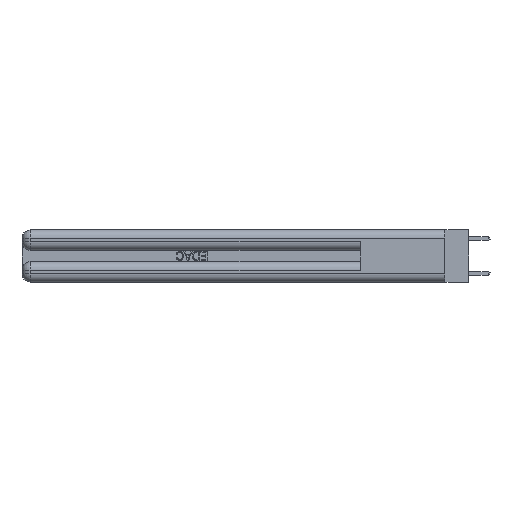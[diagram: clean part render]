
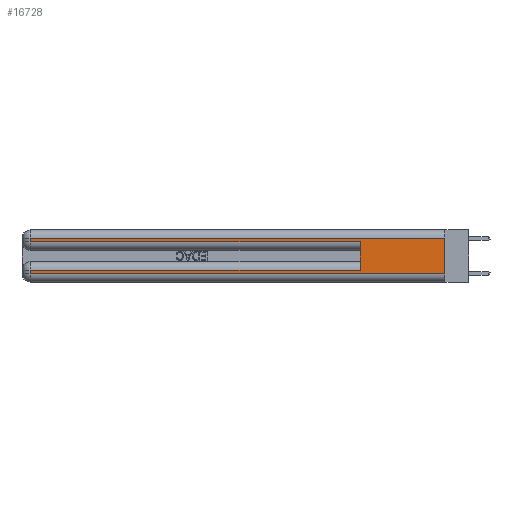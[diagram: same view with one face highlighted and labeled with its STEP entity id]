
A CAD part, left-side view. The second image highlights one B-rep face of the part: STEP entity #16728.
In plain terms, the highlighted planar face has unit normal (-1, 0, 0).
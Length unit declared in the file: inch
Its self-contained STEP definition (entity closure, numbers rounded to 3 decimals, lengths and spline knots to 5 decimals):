
#50 = CARTESIAN_POINT ( 'NONE',  ( 0., 0., 0.285 ) ) ;
#538 = DIRECTION ( 'NONE',  ( 0., 0., 1. ) ) ;
#774 = FACE_OUTER_BOUND ( 'NONE', #30095, .T. ) ;
#947 = VECTOR ( 'NONE', #8638, 39.37008 ) ;
#1196 = EDGE_CURVE ( 'NONE', #1307, #21893, #12783, .T. ) ;
#1307 = VERTEX_POINT ( 'NONE', #31573 ) ;
#3032 = CARTESIAN_POINT ( 'NONE',  ( 0., 0., 0.31 ) ) ;
#3648 = VERTEX_POINT ( 'NONE', #25622 ) ;
#3710 = CARTESIAN_POINT ( 'NONE',  ( 0., 0., 0.37 ) ) ;
#3762 = CARTESIAN_POINT ( 'NONE',  ( 0., 0.6, 0.145 ) ) ;
#4856 = EDGE_CURVE ( 'NONE', #10565, #1307, #28191, .T. ) ;
#5400 = DIRECTION ( 'NONE',  ( 1., 0., 0. ) ) ;
#6065 = CARTESIAN_POINT ( 'NONE',  ( 0., 0., 0.37 ) ) ;
#6558 = CARTESIAN_POINT ( 'NONE',  ( 0., 2.94, 0.31 ) ) ;
#6879 = CARTESIAN_POINT ( 'NONE',  ( 0., 0., 0.31 ) ) ;
#7397 = EDGE_CURVE ( 'NONE', #10565, #8087, #21836, .T. ) ;
#8087 = VERTEX_POINT ( 'NONE', #17876 ) ;
#8638 = DIRECTION ( 'NONE',  ( 0., -1., 0. ) ) ;
#9227 = ORIENTED_EDGE ( 'NONE', *, *, #4856, .T. ) ;
#10565 = VERTEX_POINT ( 'NONE', #12717 ) ;
#12412 = AXIS2_PLACEMENT_3D ( 'NONE', #6065, #5400, #16480 ) ;
#12717 = CARTESIAN_POINT ( 'NONE',  ( 0., 0.6, 0.085 ) ) ;
#12783 = LINE ( 'NONE', #18262, #14781 ) ;
#13610 = LINE ( 'NONE', #21123, #947 ) ;
#14781 = VECTOR ( 'NONE', #20474, 39.37008 ) ;
#15337 = EDGE_CURVE ( 'NONE', #31541, #3648, #23292, .T. ) ;
#15929 = CARTESIAN_POINT ( 'NONE',  ( 0., 2.94, 0.06 ) ) ;
#16176 = VECTOR ( 'NONE', #23125, 39.37008 ) ;
#16387 = EDGE_CURVE ( 'NONE', #21893, #32564, #13610, .T. ) ;
#16480 = DIRECTION ( 'NONE',  ( 0., 0., -1. ) ) ;
#16561 = CARTESIAN_POINT ( 'NONE',  ( 0., 0., 0.06 ) ) ;
#16728 = ADVANCED_FACE ( 'NONE', ( #774 ), #23965, .F. ) ;
#16973 = VECTOR ( 'NONE', #24961, 39.37008 ) ;
#17876 = CARTESIAN_POINT ( 'NONE',  ( 0., 0.6, 0.285 ) ) ;
#17976 = ORIENTED_EDGE ( 'NONE', *, *, #20560, .T. ) ;
#18227 = VECTOR ( 'NONE', #27723, 39.37008 ) ;
#18262 = CARTESIAN_POINT ( 'NONE',  ( 0., 2.94, 0.37 ) ) ;
#18801 = ORIENTED_EDGE ( 'NONE', *, *, #7397, .F. ) ;
#20187 = CARTESIAN_POINT ( 'NONE',  ( 0., 0., 0.085 ) ) ;
#20474 = DIRECTION ( 'NONE',  ( 0., 0., -1. ) ) ;
#20560 = EDGE_CURVE ( 'NONE', #21157, #31541, #27532, .T. ) ;
#20834 = LINE ( 'NONE', #50, #18227 ) ;
#20996 = ORIENTED_EDGE ( 'NONE', *, *, #15337, .T. ) ;
#21123 = CARTESIAN_POINT ( 'NONE',  ( 0., 0., 0.06 ) ) ;
#21157 = VERTEX_POINT ( 'NONE', #3032 ) ;
#21836 = LINE ( 'NONE', #3762, #29458 ) ;
#21845 = ORIENTED_EDGE ( 'NONE', *, *, #1196, .T. ) ;
#21893 = VERTEX_POINT ( 'NONE', #15929 ) ;
#22158 = ORIENTED_EDGE ( 'NONE', *, *, #16387, .T. ) ;
#22377 = ORIENTED_EDGE ( 'NONE', *, *, #31070, .F. ) ;
#23067 = DIRECTION ( 'NONE',  ( 0., 1., 0. ) ) ;
#23125 = DIRECTION ( 'NONE',  ( 0., 0., -1. ) ) ;
#23209 = ORIENTED_EDGE ( 'NONE', *, *, #24192, .T. ) ;
#23292 = LINE ( 'NONE', #33237, #16176 ) ;
#23711 = VECTOR ( 'NONE', #23067, 39.37008 ) ;
#23965 = PLANE ( 'NONE',  #12412 ) ;
#24192 = EDGE_CURVE ( 'NONE', #3648, #8087, #20834, .T. ) ;
#24327 = LINE ( 'NONE', #3710, #27140 ) ;
#24961 = DIRECTION ( 'NONE',  ( 0., 1., 0. ) ) ;
#25622 = CARTESIAN_POINT ( 'NONE',  ( 0., 2.94, 0.285 ) ) ;
#27140 = VECTOR ( 'NONE', #30150, 39.37008 ) ;
#27532 = LINE ( 'NONE', #6879, #16973 ) ;
#27723 = DIRECTION ( 'NONE',  ( 0., -1., 0. ) ) ;
#28191 = LINE ( 'NONE', #20187, #23711 ) ;
#29458 = VECTOR ( 'NONE', #538, 39.37008 ) ;
#30095 = EDGE_LOOP ( 'NONE', ( #22377, #17976, #20996, #23209, #18801, #9227, #21845, #22158 ) ) ;
#30150 = DIRECTION ( 'NONE',  ( 0., 0., -1. ) ) ;
#31070 = EDGE_CURVE ( 'NONE', #21157, #32564, #24327, .T. ) ;
#31541 = VERTEX_POINT ( 'NONE', #6558 ) ;
#31573 = CARTESIAN_POINT ( 'NONE',  ( 0., 2.94, 0.085 ) ) ;
#32564 = VERTEX_POINT ( 'NONE', #16561 ) ;
#33237 = CARTESIAN_POINT ( 'NONE',  ( 0., 2.94, 0.37 ) ) ;
